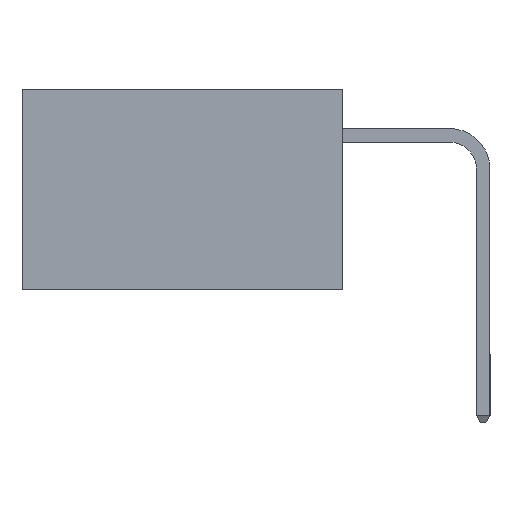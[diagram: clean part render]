
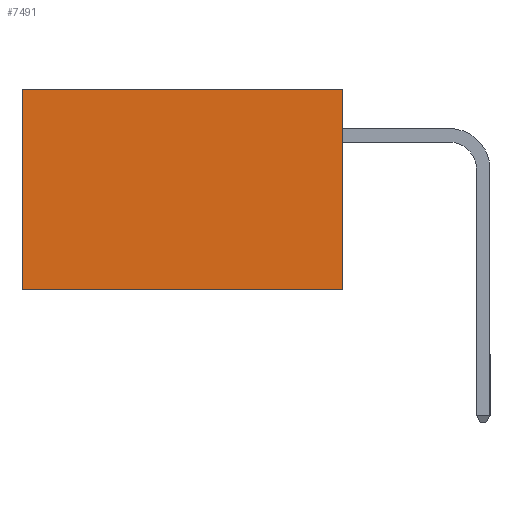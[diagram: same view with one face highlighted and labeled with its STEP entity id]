
A CAD part, left-side view. The second image highlights one B-rep face of the part: STEP entity #7491.
In plain terms, the highlighted planar face has unit normal (-1, 0, 0).
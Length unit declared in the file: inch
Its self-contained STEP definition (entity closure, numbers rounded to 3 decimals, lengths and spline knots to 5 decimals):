
#302 = ORIENTED_EDGE ( 'NONE', *, *, #21272, .F. ) ;
#463 = PLANE ( 'NONE',  #26020 ) ;
#1341 = CARTESIAN_POINT ( 'NONE',  ( 0.277, 0., 0. ) ) ;
#1817 = VECTOR ( 'NONE', #2887, 39.37008 ) ;
#2517 = DIRECTION ( 'NONE',  ( 0., 0., -1. ) ) ;
#2887 = DIRECTION ( 'NONE',  ( 0., 1., 0. ) ) ;
#3226 = CARTESIAN_POINT ( 'NONE',  ( 0.277, 0., -0.37 ) ) ;
#3559 = LINE ( 'NONE', #15811, #24514 ) ;
#4077 = ORIENTED_EDGE ( 'NONE', *, *, #13353, .T. ) ;
#4079 = CARTESIAN_POINT ( 'NONE',  ( 0.277, 0.59, 0. ) ) ;
#4206 = FACE_OUTER_BOUND ( 'NONE', #17951, .T. ) ;
#4309 = VERTEX_POINT ( 'NONE', #7479 ) ;
#6590 = LINE ( 'NONE', #15044, #1817 ) ;
#6749 = VERTEX_POINT ( 'NONE', #4079 ) ;
#7309 = CARTESIAN_POINT ( 'NONE',  ( 0.277, 0.59, -0.37 ) ) ;
#7479 = CARTESIAN_POINT ( 'NONE',  ( 0.277, 0., -0.37 ) ) ;
#7491 = ADVANCED_FACE ( 'NONE', ( #4206 ), #463, .F. ) ;
#9174 = CARTESIAN_POINT ( 'NONE',  ( 0.277, 0.59, -0.37 ) ) ;
#9782 = VERTEX_POINT ( 'NONE', #1341 ) ;
#13353 = EDGE_CURVE ( 'NONE', #6749, #23672, #16451, .T. ) ;
#14336 = ORIENTED_EDGE ( 'NONE', *, *, #20416, .F. ) ;
#14550 = ORIENTED_EDGE ( 'NONE', *, *, #25101, .T. ) ;
#14676 = DIRECTION ( 'NONE',  ( 1., 0., 0. ) ) ;
#15044 = CARTESIAN_POINT ( 'NONE',  ( 0.277, 0., 0. ) ) ;
#15811 = CARTESIAN_POINT ( 'NONE',  ( 0.277, 0., -0.37 ) ) ;
#15903 = DIRECTION ( 'NONE',  ( 0., 0., -1. ) ) ;
#16451 = LINE ( 'NONE', #7309, #23097 ) ;
#17456 = DIRECTION ( 'NONE',  ( 0., 1., 0. ) ) ;
#17951 = EDGE_LOOP ( 'NONE', ( #4077, #14336, #302, #14550 ) ) ;
#19827 = VECTOR ( 'NONE', #17456, 39.37008 ) ;
#20416 = EDGE_CURVE ( 'NONE', #4309, #23672, #24573, .T. ) ;
#20750 = CARTESIAN_POINT ( 'NONE',  ( 0.277, 0., -0.37 ) ) ;
#21272 = EDGE_CURVE ( 'NONE', #9782, #4309, #3559, .T. ) ;
#23097 = VECTOR ( 'NONE', #23545, 39.37008 ) ;
#23545 = DIRECTION ( 'NONE',  ( 0., 0., -1. ) ) ;
#23672 = VERTEX_POINT ( 'NONE', #9174 ) ;
#24514 = VECTOR ( 'NONE', #15903, 39.37008 ) ;
#24573 = LINE ( 'NONE', #3226, #19827 ) ;
#25101 = EDGE_CURVE ( 'NONE', #9782, #6749, #6590, .T. ) ;
#26020 = AXIS2_PLACEMENT_3D ( 'NONE', #20750, #14676, #2517 ) ;
